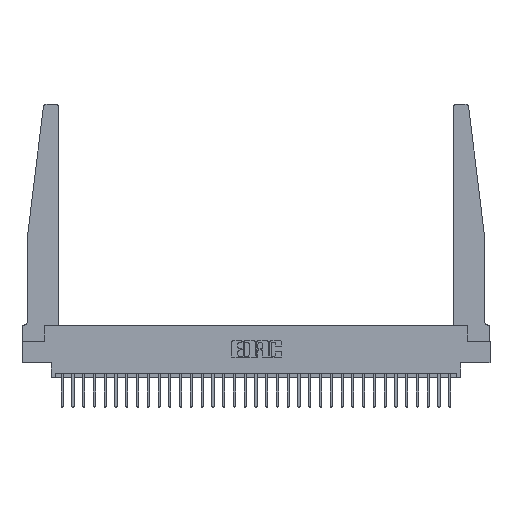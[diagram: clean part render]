
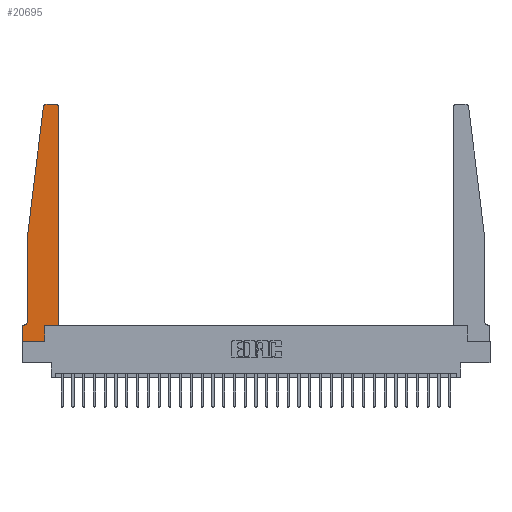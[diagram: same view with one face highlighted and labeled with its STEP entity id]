
A CAD part, top view. The second image highlights one B-rep face of the part: STEP entity #20695.
In plain terms, the highlighted planar face has unit normal (0, 0, 1).
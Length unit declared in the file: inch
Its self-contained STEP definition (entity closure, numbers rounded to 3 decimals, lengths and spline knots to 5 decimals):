
#206 = LINE ( 'NONE', #9543, #4936 ) ;
#289 = VERTEX_POINT ( 'NONE', #929 ) ;
#717 = CIRCLE ( 'NONE', #26567, 0.03 ) ;
#929 = CARTESIAN_POINT ( 'NONE',  ( 0.065, 0.2375, 0.37 ) ) ;
#2124 = CARTESIAN_POINT ( 'NONE',  ( 0., 0., 0.37 ) ) ;
#2152 = LINE ( 'NONE', #27956, #28184 ) ;
#2926 = LINE ( 'NONE', #4917, #28831 ) ;
#2970 = LINE ( 'NONE', #3421, #10304 ) ;
#3407 = VERTEX_POINT ( 'NONE', #18560 ) ;
#3421 = CARTESIAN_POINT ( 'NONE',  ( 0.065, 0.1875, 0.37 ) ) ;
#3581 = EDGE_CURVE ( 'NONE', #4808, #10339, #12005, .T. ) ;
#4067 = AXIS2_PLACEMENT_3D ( 'NONE', #11155, #30084, #4114 ) ;
#4074 = ORIENTED_EDGE ( 'NONE', *, *, #15909, .T. ) ;
#4114 = DIRECTION ( 'NONE',  ( 1., 0., 0. ) ) ;
#4183 = VERTEX_POINT ( 'NONE', #9181 ) ;
#4808 = VERTEX_POINT ( 'NONE', #12053 ) ;
#4894 = CARTESIAN_POINT ( 'NONE',  ( 0.24675, 2.72367, 0.37 ) ) ;
#4917 = CARTESIAN_POINT ( 'NONE',  ( 0.425, 0.18, 0.37 ) ) ;
#4936 = VECTOR ( 'NONE', #28170, 39.37008 ) ;
#6094 = CIRCLE ( 'NONE', #11537, 0.05 ) ;
#6238 = DIRECTION ( 'NONE',  ( 0., -1., 0. ) ) ;
#6406 = FACE_OUTER_BOUND ( 'NONE', #21750, .T. ) ;
#6415 = VERTEX_POINT ( 'NONE', #21691 ) ;
#6808 = DIRECTION ( 'NONE',  ( 0., 0., -1. ) ) ;
#7468 = ORIENTED_EDGE ( 'NONE', *, *, #3581, .T. ) ;
#7703 = ORIENTED_EDGE ( 'NONE', *, *, #16272, .T. ) ;
#8055 = CIRCLE ( 'NONE', #15350, 0.03 ) ;
#8375 = LINE ( 'NONE', #13418, #23109 ) ;
#8475 = VERTEX_POINT ( 'NONE', #10319 ) ;
#8801 = CARTESIAN_POINT ( 'NONE',  ( 0.425, 0.18, 0.37 ) ) ;
#9181 = CARTESIAN_POINT ( 'NONE',  ( 0., 0.1875, 0.37 ) ) ;
#9420 = VERTEX_POINT ( 'NONE', #4894 ) ;
#9543 = CARTESIAN_POINT ( 'NONE',  ( 0., 0., 0.37 ) ) ;
#9559 = DIRECTION ( 'NONE',  ( 1., 0., 0. ) ) ;
#9764 = EDGE_CURVE ( 'NONE', #15026, #289, #8375, .T. ) ;
#9951 = CARTESIAN_POINT ( 'NONE',  ( 0.065, 1.25, 0.37 ) ) ;
#10304 = VECTOR ( 'NONE', #26796, 39.37008 ) ;
#10319 = CARTESIAN_POINT ( 'NONE',  ( 0.27653, 2.75, 0.37 ) ) ;
#10339 = VERTEX_POINT ( 'NONE', #8801 ) ;
#10810 = CARTESIAN_POINT ( 'NONE',  ( 0.25, 2.75, 0.37 ) ) ;
#11155 = CARTESIAN_POINT ( 'NONE',  ( 0., 0.1875, 0.37 ) ) ;
#11265 = DIRECTION ( 'NONE',  ( -1., 0., 0. ) ) ;
#11537 = AXIS2_PLACEMENT_3D ( 'NONE', #25596, #6808, #11562 ) ;
#11562 = DIRECTION ( 'NONE',  ( -1., 0., 0. ) ) ;
#11644 = EDGE_CURVE ( 'NONE', #289, #20468, #6094, .T. ) ;
#11849 = DIRECTION ( 'NONE',  ( 0., 0., 1. ) ) ;
#12005 = LINE ( 'NONE', #14581, #16270 ) ;
#12053 = CARTESIAN_POINT ( 'NONE',  ( 0.2605, 0.18, 0.37 ) ) ;
#12523 = EDGE_CURVE ( 'NONE', #9420, #15026, #2152, .T. ) ;
#13037 = ORIENTED_EDGE ( 'NONE', *, *, #22641, .T. ) ;
#13255 = VECTOR ( 'NONE', #11265, 39.37008 ) ;
#13418 = CARTESIAN_POINT ( 'NONE',  ( 0.065, 1.25, 0.37 ) ) ;
#13618 = DIRECTION ( 'NONE',  ( -0.122, -0.992, 0. ) ) ;
#13928 = DIRECTION ( 'NONE',  ( 0., 0., 1. ) ) ;
#14581 = CARTESIAN_POINT ( 'NONE',  ( 0.425, 0.18, 0.37 ) ) ;
#14730 = CARTESIAN_POINT ( 'NONE',  ( 0.2605, 0.18, 0.37 ) ) ;
#15026 = VERTEX_POINT ( 'NONE', #9951 ) ;
#15350 = AXIS2_PLACEMENT_3D ( 'NONE', #23153, #11849, #9559 ) ;
#15721 = PLANE ( 'NONE',  #4067 ) ;
#15758 = CARTESIAN_POINT ( 'NONE',  ( 0.27653, 2.72, 0.37 ) ) ;
#15909 = EDGE_CURVE ( 'NONE', #4183, #20768, #206, .T. ) ;
#16270 = VECTOR ( 'NONE', #23902, 39.37008 ) ;
#16272 = EDGE_CURVE ( 'NONE', #10339, #3407, #2926, .T. ) ;
#16526 = CARTESIAN_POINT ( 'NONE',  ( 0.015, 0.1875, 0.37 ) ) ;
#16621 = EDGE_CURVE ( 'NONE', #20768, #6415, #20462, .T. ) ;
#17025 = EDGE_CURVE ( 'NONE', #22952, #8475, #20429, .T. ) ;
#18028 = DIRECTION ( 'NONE',  ( 1., 0., 0. ) ) ;
#18560 = CARTESIAN_POINT ( 'NONE',  ( 0.425, 2.72, 0.37 ) ) ;
#19307 = ORIENTED_EDGE ( 'NONE', *, *, #25406, .T. ) ;
#19315 = ORIENTED_EDGE ( 'NONE', *, *, #12523, .T. ) ;
#20280 = EDGE_CURVE ( 'NONE', #8475, #9420, #717, .T. ) ;
#20429 = LINE ( 'NONE', #10810, #13255 ) ;
#20462 = LINE ( 'NONE', #2124, #22499 ) ;
#20468 = VERTEX_POINT ( 'NONE', #16526 ) ;
#20695 = ADVANCED_FACE ( 'NONE', ( #6406 ), #15721, .T. ) ;
#20768 = VERTEX_POINT ( 'NONE', #27473 ) ;
#21526 = ORIENTED_EDGE ( 'NONE', *, *, #17025, .T. ) ;
#21553 = DIRECTION ( 'NONE',  ( 0., 1., 0. ) ) ;
#21691 = CARTESIAN_POINT ( 'NONE',  ( 0.2605, 0., 0.37 ) ) ;
#21750 = EDGE_LOOP ( 'NONE', ( #21526, #21835, #19315, #22648, #28515, #22659, #4074, #26855, #19307, #7468, #7703, #13037 ) ) ;
#21835 = ORIENTED_EDGE ( 'NONE', *, *, #20280, .T. ) ;
#22499 = VECTOR ( 'NONE', #18028, 39.37008 ) ;
#22641 = EDGE_CURVE ( 'NONE', #3407, #22952, #8055, .T. ) ;
#22648 = ORIENTED_EDGE ( 'NONE', *, *, #9764, .T. ) ;
#22659 = ORIENTED_EDGE ( 'NONE', *, *, #27962, .T. ) ;
#22952 = VERTEX_POINT ( 'NONE', #22955 ) ;
#22955 = CARTESIAN_POINT ( 'NONE',  ( 0.395, 2.75, 0.37 ) ) ;
#23109 = VECTOR ( 'NONE', #6238, 39.37008 ) ;
#23153 = CARTESIAN_POINT ( 'NONE',  ( 0.395, 2.72, 0.37 ) ) ;
#23270 = VECTOR ( 'NONE', #29378, 39.37008 ) ;
#23902 = DIRECTION ( 'NONE',  ( 1., 0., 0. ) ) ;
#25406 = EDGE_CURVE ( 'NONE', #6415, #4808, #29237, .T. ) ;
#25596 = CARTESIAN_POINT ( 'NONE',  ( 0.015, 0.2375, 0.37 ) ) ;
#26567 = AXIS2_PLACEMENT_3D ( 'NONE', #15758, #13928, #29972 ) ;
#26796 = DIRECTION ( 'NONE',  ( -1., 0., 0. ) ) ;
#26855 = ORIENTED_EDGE ( 'NONE', *, *, #16621, .T. ) ;
#27473 = CARTESIAN_POINT ( 'NONE',  ( 0., 0., 0.37 ) ) ;
#27956 = CARTESIAN_POINT ( 'NONE',  ( 0.065, 1.25, 0.37 ) ) ;
#27962 = EDGE_CURVE ( 'NONE', #20468, #4183, #2970, .T. ) ;
#28170 = DIRECTION ( 'NONE',  ( 0., -1., 0. ) ) ;
#28184 = VECTOR ( 'NONE', #13618, 39.37008 ) ;
#28515 = ORIENTED_EDGE ( 'NONE', *, *, #11644, .T. ) ;
#28831 = VECTOR ( 'NONE', #21553, 39.37008 ) ;
#29237 = LINE ( 'NONE', #14730, #23270 ) ;
#29378 = DIRECTION ( 'NONE',  ( 0., 1., 0. ) ) ;
#29972 = DIRECTION ( 'NONE',  ( 1., 0., 0. ) ) ;
#30084 = DIRECTION ( 'NONE',  ( 0., 0., 1. ) ) ;
